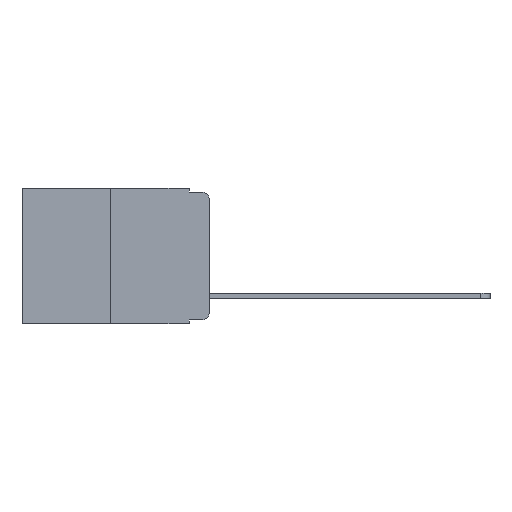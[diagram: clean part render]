
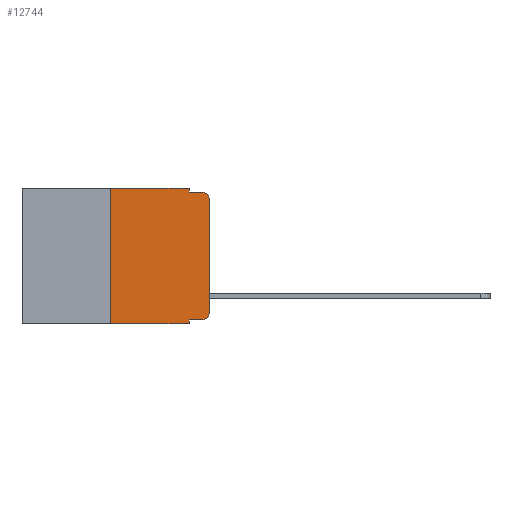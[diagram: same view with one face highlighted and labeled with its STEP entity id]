
A CAD part, left-side view. The second image highlights one B-rep face of the part: STEP entity #12744.
In plain terms, the highlighted planar face has unit normal (-1, 0, 0).
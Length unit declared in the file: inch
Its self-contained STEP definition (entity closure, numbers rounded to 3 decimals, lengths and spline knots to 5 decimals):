
#166 = DIRECTION ( 'NONE',  ( 0., -1., 0. ) ) ;
#233 = LINE ( 'NONE', #4957, #1029 ) ;
#244 = ORIENTED_EDGE ( 'NONE', *, *, #8167, .T. ) ;
#410 = DIRECTION ( 'NONE',  ( 0., 0., 1. ) ) ;
#418 = ORIENTED_EDGE ( 'NONE', *, *, #14582, .T. ) ;
#581 = CARTESIAN_POINT ( 'NONE',  ( 0., 0.051, 0. ) ) ;
#760 = DIRECTION ( 'NONE',  ( 0., 0., -1. ) ) ;
#822 = AXIS2_PLACEMENT_3D ( 'NONE', #5212, #13054, #6414 ) ;
#1022 = ORIENTED_EDGE ( 'NONE', *, *, #4203, .T. ) ;
#1029 = VECTOR ( 'NONE', #1273, 39.37008 ) ;
#1165 = ORIENTED_EDGE ( 'NONE', *, *, #1913, .F. ) ;
#1208 = LINE ( 'NONE', #2678, #6583 ) ;
#1273 = DIRECTION ( 'NONE',  ( 0., 0., 1. ) ) ;
#1498 = VERTEX_POINT ( 'NONE', #3849 ) ;
#1546 = DIRECTION ( 'NONE',  ( 1., 0., 0. ) ) ;
#1645 = CARTESIAN_POINT ( 'NONE',  ( 0., 0.473, 0. ) ) ;
#1913 = EDGE_CURVE ( 'NONE', #7873, #1498, #10478, .T. ) ;
#1948 = VERTEX_POINT ( 'NONE', #5949 ) ;
#2159 = EDGE_CURVE ( 'NONE', #1948, #7873, #1208, .T. ) ;
#2611 = LINE ( 'NONE', #9317, #5534 ) ;
#2678 = CARTESIAN_POINT ( 'NONE',  ( 0., 0.051, 0. ) ) ;
#2705 = VECTOR ( 'NONE', #410, 39.37008 ) ;
#3043 = VERTEX_POINT ( 'NONE', #10801 ) ;
#3566 = ORIENTED_EDGE ( 'NONE', *, *, #6347, .T. ) ;
#3607 = ORIENTED_EDGE ( 'NONE', *, *, #9031, .T. ) ;
#3615 = CARTESIAN_POINT ( 'NONE',  ( 0., 0.051, -0.343 ) ) ;
#3817 = AXIS2_PLACEMENT_3D ( 'NONE', #9781, #1546, #9831 ) ;
#3832 = VERTEX_POINT ( 'NONE', #8492 ) ;
#3849 = CARTESIAN_POINT ( 'NONE',  ( 0., 0.02, -0.01 ) ) ;
#3860 = ORIENTED_EDGE ( 'NONE', *, *, #7864, .F. ) ;
#4168 = VERTEX_POINT ( 'NONE', #3615 ) ;
#4203 = EDGE_CURVE ( 'NONE', #4217, #3043, #8676, .T. ) ;
#4217 = VERTEX_POINT ( 'NONE', #7055 ) ;
#4579 = DIRECTION ( 'NONE',  ( 0., -1., 0. ) ) ;
#4957 = CARTESIAN_POINT ( 'NONE',  ( 0., 0.25, 0. ) ) ;
#5008 = EDGE_LOOP ( 'NONE', ( #1022, #3566, #1165, #11344, #3860, #6709, #244, #14448, #3607, #418 ) ) ;
#5212 = CARTESIAN_POINT ( 'NONE',  ( 0., 0.02, -0.313 ) ) ;
#5534 = VECTOR ( 'NONE', #10462, 39.37008 ) ;
#5696 = VERTEX_POINT ( 'NONE', #8954 ) ;
#5949 = CARTESIAN_POINT ( 'NONE',  ( 0., 0.051, 0. ) ) ;
#6025 = CIRCLE ( 'NONE', #822, 0.02 ) ;
#6347 = EDGE_CURVE ( 'NONE', #3043, #1498, #10722, .T. ) ;
#6414 = DIRECTION ( 'NONE',  ( 0., 0., -1. ) ) ;
#6434 = PLANE ( 'NONE',  #3817 ) ;
#6452 = CARTESIAN_POINT ( 'NONE',  ( 0., 0.02, -0.333 ) ) ;
#6583 = VECTOR ( 'NONE', #760, 39.37008 ) ;
#6706 = CARTESIAN_POINT ( 'NONE',  ( 0., 0.02, -0.03 ) ) ;
#6709 = ORIENTED_EDGE ( 'NONE', *, *, #8945, .F. ) ;
#6766 = VERTEX_POINT ( 'NONE', #11911 ) ;
#6840 = VERTEX_POINT ( 'NONE', #6452 ) ;
#7055 = CARTESIAN_POINT ( 'NONE',  ( 0., 0., -0.313 ) ) ;
#7169 = LINE ( 'NONE', #1645, #10532 ) ;
#7347 = AXIS2_PLACEMENT_3D ( 'NONE', #6706, #14398, #7851 ) ;
#7851 = DIRECTION ( 'NONE',  ( 0., 0., -1. ) ) ;
#7864 = EDGE_CURVE ( 'NONE', #5696, #1948, #7169, .T. ) ;
#7873 = VERTEX_POINT ( 'NONE', #13209 ) ;
#8167 = EDGE_CURVE ( 'NONE', #3832, #4168, #2611, .T. ) ;
#8366 = VECTOR ( 'NONE', #166, 39.37008 ) ;
#8492 = CARTESIAN_POINT ( 'NONE',  ( 0., 0.25, -0.343 ) ) ;
#8676 = LINE ( 'NONE', #11514, #2705 ) ;
#8791 = DIRECTION ( 'NONE',  ( 0., -1., 0. ) ) ;
#8945 = EDGE_CURVE ( 'NONE', #3832, #5696, #233, .T. ) ;
#8953 = FACE_OUTER_BOUND ( 'NONE', #5008, .T. ) ;
#8954 = CARTESIAN_POINT ( 'NONE',  ( 0., 0.25, 0. ) ) ;
#9031 = EDGE_CURVE ( 'NONE', #6766, #6840, #12699, .T. ) ;
#9317 = CARTESIAN_POINT ( 'NONE',  ( 0., 0.473, -0.343 ) ) ;
#9781 = CARTESIAN_POINT ( 'NONE',  ( 0., 0.473, 0. ) ) ;
#9831 = DIRECTION ( 'NONE',  ( 0., 0., -1. ) ) ;
#9927 = LINE ( 'NONE', #581, #11835 ) ;
#10123 = VECTOR ( 'NONE', #4579, 39.37008 ) ;
#10462 = DIRECTION ( 'NONE',  ( 0., -1., 0. ) ) ;
#10478 = LINE ( 'NONE', #11288, #10123 ) ;
#10532 = VECTOR ( 'NONE', #8791, 39.37008 ) ;
#10722 = CIRCLE ( 'NONE', #7347, 0.02 ) ;
#10801 = CARTESIAN_POINT ( 'NONE',  ( 0., 0., -0.03 ) ) ;
#11288 = CARTESIAN_POINT ( 'NONE',  ( 0., 0.051, -0.01 ) ) ;
#11344 = ORIENTED_EDGE ( 'NONE', *, *, #2159, .F. ) ;
#11514 = CARTESIAN_POINT ( 'NONE',  ( 0., 0., 0. ) ) ;
#11835 = VECTOR ( 'NONE', #12320, 39.37008 ) ;
#11911 = CARTESIAN_POINT ( 'NONE',  ( 0., 0.051, -0.333 ) ) ;
#11944 = CARTESIAN_POINT ( 'NONE',  ( 0., 0.051, -0.333 ) ) ;
#12320 = DIRECTION ( 'NONE',  ( 0., 0., -1. ) ) ;
#12699 = LINE ( 'NONE', #11944, #8366 ) ;
#12744 = ADVANCED_FACE ( 'NONE', ( #8953 ), #6434, .F. ) ;
#13054 = DIRECTION ( 'NONE',  ( -1., 0., 0. ) ) ;
#13209 = CARTESIAN_POINT ( 'NONE',  ( 0., 0.051, -0.01 ) ) ;
#14398 = DIRECTION ( 'NONE',  ( -1., 0., 0. ) ) ;
#14448 = ORIENTED_EDGE ( 'NONE', *, *, #14749, .F. ) ;
#14582 = EDGE_CURVE ( 'NONE', #6840, #4217, #6025, .T. ) ;
#14749 = EDGE_CURVE ( 'NONE', #6766, #4168, #9927, .T. ) ;
